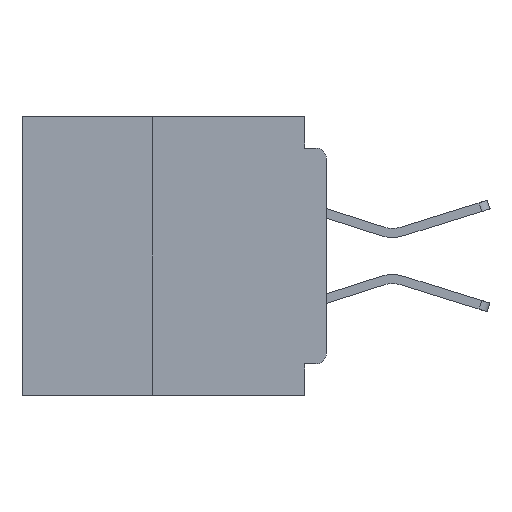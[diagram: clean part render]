
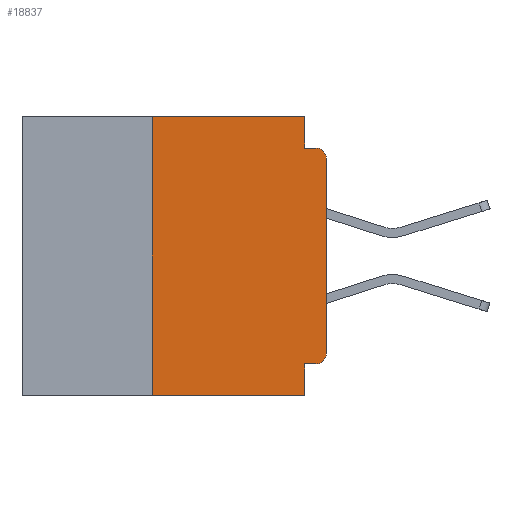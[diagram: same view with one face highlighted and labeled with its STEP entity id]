
A CAD part, left-side view. The second image highlights one B-rep face of the part: STEP entity #18837.
In plain terms, the highlighted planar face has unit normal (-1, 0, 0).
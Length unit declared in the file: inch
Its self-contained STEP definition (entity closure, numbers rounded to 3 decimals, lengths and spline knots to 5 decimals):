
#223 = LINE ( 'NONE', #44396, #29032 ) ;
#888 = ORIENTED_EDGE ( 'NONE', *, *, #27729, .T. ) ;
#1656 = CARTESIAN_POINT ( 'NONE',  ( 0., 0.437, 0. ) ) ;
#1848 = VERTEX_POINT ( 'NONE', #33962 ) ;
#3314 = DIRECTION ( 'NONE',  ( 0., 0., 1. ) ) ;
#3652 = AXIS2_PLACEMENT_3D ( 'NONE', #42512, #20883, #46123 ) ;
#3799 = VERTEX_POINT ( 'NONE', #23984 ) ;
#4243 = VECTOR ( 'NONE', #24436, 39.37008 ) ;
#4814 = ORIENTED_EDGE ( 'NONE', *, *, #14649, .T. ) ;
#5302 = DIRECTION ( 'NONE',  ( 0., 0., -1. ) ) ;
#5505 = CARTESIAN_POINT ( 'NONE',  ( 0., 0.031, -0.355 ) ) ;
#5507 = ORIENTED_EDGE ( 'NONE', *, *, #14670, .F. ) ;
#6867 = AXIS2_PLACEMENT_3D ( 'NONE', #30617, #8958, #34246 ) ;
#7831 = EDGE_CURVE ( 'NONE', #3799, #23052, #44201, .T. ) ;
#8958 = DIRECTION ( 'NONE',  ( -1., 0., 0. ) ) ;
#9052 = VERTEX_POINT ( 'NONE', #5505 ) ;
#9503 = DIRECTION ( 'NONE',  ( 0., -1., 0. ) ) ;
#10220 = ORIENTED_EDGE ( 'NONE', *, *, #34908, .F. ) ;
#10810 = VERTEX_POINT ( 'NONE', #37904 ) ;
#11436 = EDGE_CURVE ( 'NONE', #10810, #33305, #36027, .T. ) ;
#12591 = CARTESIAN_POINT ( 'NONE',  ( 0., 0.031, 0. ) ) ;
#13314 = VECTOR ( 'NONE', #41409, 39.37008 ) ;
#13515 = CARTESIAN_POINT ( 'NONE',  ( 0., 0.031, -0.4 ) ) ;
#13847 = LINE ( 'NONE', #13515, #4243 ) ;
#14347 = VERTEX_POINT ( 'NONE', #29047 ) ;
#14649 = EDGE_CURVE ( 'NONE', #23052, #1848, #25261, .T. ) ;
#14670 = EDGE_CURVE ( 'NONE', #32432, #14347, #44464, .T. ) ;
#16522 = DIRECTION ( 'NONE',  ( 0., 0., 1. ) ) ;
#16615 = CARTESIAN_POINT ( 'NONE',  ( 0., 0.015, -0.355 ) ) ;
#17199 = ORIENTED_EDGE ( 'NONE', *, *, #18147, .F. ) ;
#17471 = EDGE_LOOP ( 'NONE', ( #33829, #4814, #30598, #5507, #10220, #38876, #45702, #32186, #17199, #888 ) ) ;
#18147 = EDGE_CURVE ( 'NONE', #39553, #9052, #26032, .T. ) ;
#18837 = ADVANCED_FACE ( 'NONE', ( #42974 ), #26627, .F. ) ;
#19790 = CARTESIAN_POINT ( 'NONE',  ( 0., 0.437, 0. ) ) ;
#19878 = CARTESIAN_POINT ( 'NONE',  ( 0., 0.031, -0.4 ) ) ;
#20883 = DIRECTION ( 'NONE',  ( -1., 0., 0. ) ) ;
#22765 = DIRECTION ( 'NONE',  ( 0., -1., 0. ) ) ;
#23052 = VERTEX_POINT ( 'NONE', #37398 ) ;
#23338 = AXIS2_PLACEMENT_3D ( 'NONE', #1656, #26938, #5302 ) ;
#23984 = CARTESIAN_POINT ( 'NONE',  ( 0., 0., -0.34 ) ) ;
#24077 = CIRCLE ( 'NONE', #3652, 0.015 ) ;
#24115 = VECTOR ( 'NONE', #26983, 39.37008 ) ;
#24436 = DIRECTION ( 'NONE',  ( 0., 0., -1. ) ) ;
#25261 = CIRCLE ( 'NONE', #6867, 0.015 ) ;
#26032 = LINE ( 'NONE', #41210, #42965 ) ;
#26627 = PLANE ( 'NONE',  #23338 ) ;
#26938 = DIRECTION ( 'NONE',  ( 1., 0., 0. ) ) ;
#26983 = DIRECTION ( 'NONE',  ( 0., 0., -1. ) ) ;
#27729 = EDGE_CURVE ( 'NONE', #39553, #3799, #24077, .T. ) ;
#28943 = VERTEX_POINT ( 'NONE', #19878 ) ;
#29032 = VECTOR ( 'NONE', #22765, 39.37008 ) ;
#29047 = CARTESIAN_POINT ( 'NONE',  ( 0., 0.031, -0.045 ) ) ;
#30598 = ORIENTED_EDGE ( 'NONE', *, *, #44800, .F. ) ;
#30617 = CARTESIAN_POINT ( 'NONE',  ( 0., 0.015, -0.06 ) ) ;
#31145 = CARTESIAN_POINT ( 'NONE',  ( 0., 0., -0.045 ) ) ;
#31904 = VECTOR ( 'NONE', #9503, 39.37008 ) ;
#32186 = ORIENTED_EDGE ( 'NONE', *, *, #40984, .F. ) ;
#32432 = VERTEX_POINT ( 'NONE', #46069 ) ;
#32590 = LINE ( 'NONE', #19790, #13314 ) ;
#33088 = CARTESIAN_POINT ( 'NONE',  ( 0., 0.25, 0. ) ) ;
#33305 = VERTEX_POINT ( 'NONE', #33088 ) ;
#33829 = ORIENTED_EDGE ( 'NONE', *, *, #7831, .T. ) ;
#33962 = CARTESIAN_POINT ( 'NONE',  ( 0., 0.015, -0.045 ) ) ;
#34246 = DIRECTION ( 'NONE',  ( 0., 0., -1. ) ) ;
#34908 = EDGE_CURVE ( 'NONE', #33305, #32432, #32590, .T. ) ;
#35726 = VECTOR ( 'NONE', #16522, 39.37008 ) ;
#36027 = LINE ( 'NONE', #46552, #46715 ) ;
#37398 = CARTESIAN_POINT ( 'NONE',  ( 0., 0., -0.06 ) ) ;
#37604 = DIRECTION ( 'NONE',  ( 0., 1., 0. ) ) ;
#37904 = CARTESIAN_POINT ( 'NONE',  ( 0., 0.25, -0.4 ) ) ;
#38172 = CARTESIAN_POINT ( 'NONE',  ( 0., 0., 0. ) ) ;
#38876 = ORIENTED_EDGE ( 'NONE', *, *, #11436, .F. ) ;
#39553 = VERTEX_POINT ( 'NONE', #16615 ) ;
#40984 = EDGE_CURVE ( 'NONE', #9052, #28943, #13847, .T. ) ;
#41210 = CARTESIAN_POINT ( 'NONE',  ( 0., 0., -0.355 ) ) ;
#41409 = DIRECTION ( 'NONE',  ( 0., -1., 0. ) ) ;
#41509 = LINE ( 'NONE', #31145, #31904 ) ;
#42512 = CARTESIAN_POINT ( 'NONE',  ( 0., 0.015, -0.34 ) ) ;
#42965 = VECTOR ( 'NONE', #37604, 39.37008 ) ;
#42974 = FACE_OUTER_BOUND ( 'NONE', #17471, .T. ) ;
#44201 = LINE ( 'NONE', #38172, #35726 ) ;
#44396 = CARTESIAN_POINT ( 'NONE',  ( 0., 0.437, -0.4 ) ) ;
#44464 = LINE ( 'NONE', #12591, #24115 ) ;
#44800 = EDGE_CURVE ( 'NONE', #14347, #1848, #41509, .T. ) ;
#45132 = EDGE_CURVE ( 'NONE', #10810, #28943, #223, .T. ) ;
#45702 = ORIENTED_EDGE ( 'NONE', *, *, #45132, .T. ) ;
#46069 = CARTESIAN_POINT ( 'NONE',  ( 0., 0.031, 0. ) ) ;
#46123 = DIRECTION ( 'NONE',  ( 0., 0., -1. ) ) ;
#46552 = CARTESIAN_POINT ( 'NONE',  ( 0., 0.25, -0.4 ) ) ;
#46715 = VECTOR ( 'NONE', #3314, 39.37008 ) ;
